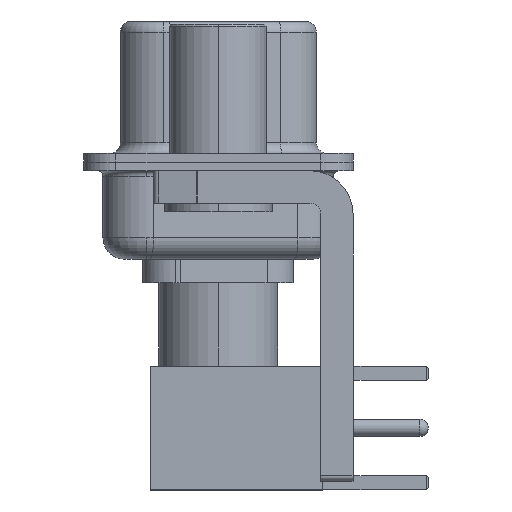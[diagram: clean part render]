
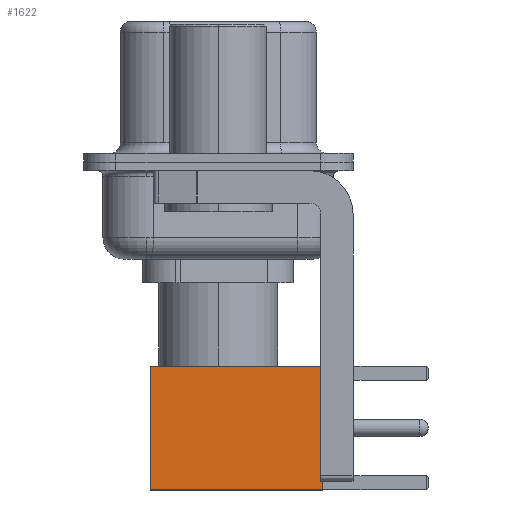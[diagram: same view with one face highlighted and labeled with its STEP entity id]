
A CAD part, left-side view. The second image highlights one B-rep face of the part: STEP entity #1622.
In plain terms, the highlighted face is planar.
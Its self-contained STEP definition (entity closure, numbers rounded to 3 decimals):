
#90 = ORIENTED_EDGE ( 'NONE', *, *, #21384, .F. ) ;
#355 = VERTEX_POINT ( 'NONE', #14789 ) ;
#576 = AXIS2_PLACEMENT_3D ( 'NONE', #3930, #20955, #12417 ) ;
#872 = CARTESIAN_POINT ( 'NONE',  ( -2.875, 2.875, 8. ) ) ;
#1123 = ORIENTED_EDGE ( 'NONE', *, *, #7999, .T. ) ;
#1265 = CARTESIAN_POINT ( 'NONE',  ( -2.875, 2.875, 0. ) ) ;
#1622 = ADVANCED_FACE ( 'NONE', ( #5616 ), #19503, .T. ) ;
#2827 = VECTOR ( 'NONE', #21003, 1000. ) ;
#3165 = CARTESIAN_POINT ( 'NONE',  ( 2.875, 2.875, 8. ) ) ;
#3533 = VERTEX_POINT ( 'NONE', #3165 ) ;
#3930 = CARTESIAN_POINT ( 'NONE',  ( 2.875, 2.875, 0. ) ) ;
#4391 = VERTEX_POINT ( 'NONE', #872 ) ;
#4683 = DIRECTION ( 'NONE',  ( -1., 0., 0. ) ) ;
#4715 = CARTESIAN_POINT ( 'NONE',  ( -2.875, 2.875, 0. ) ) ;
#5616 = FACE_OUTER_BOUND ( 'NONE', #14659, .T. ) ;
#6044 = LINE ( 'NONE', #6254, #14797 ) ;
#6254 = CARTESIAN_POINT ( 'NONE',  ( 0., 2.875, 8. ) ) ;
#6876 = CARTESIAN_POINT ( 'NONE',  ( 2.875, 2.875, 0. ) ) ;
#7000 = LINE ( 'NONE', #14170, #2827 ) ;
#7999 = EDGE_CURVE ( 'NONE', #355, #9861, #7000, .T. ) ;
#8033 = EDGE_CURVE ( 'NONE', #4391, #9861, #21232, .T. ) ;
#9861 = VERTEX_POINT ( 'NONE', #1265 ) ;
#10305 = VECTOR ( 'NONE', #13447, 1000. ) ;
#11564 = LINE ( 'NONE', #6876, #14530 ) ;
#12417 = DIRECTION ( 'NONE',  ( 0., 0., 1. ) ) ;
#12677 = EDGE_CURVE ( 'NONE', #3533, #355, #11564, .T. ) ;
#13447 = DIRECTION ( 'NONE',  ( 0., 0., -1. ) ) ;
#14170 = CARTESIAN_POINT ( 'NONE',  ( 0., 2.875, 0. ) ) ;
#14530 = VECTOR ( 'NONE', #20555, 1000. ) ;
#14659 = EDGE_LOOP ( 'NONE', ( #21612, #1123, #15480, #90 ) ) ;
#14789 = CARTESIAN_POINT ( 'NONE',  ( 2.875, 2.875, 0. ) ) ;
#14797 = VECTOR ( 'NONE', #4683, 1000. ) ;
#15480 = ORIENTED_EDGE ( 'NONE', *, *, #8033, .F. ) ;
#19503 = PLANE ( 'NONE',  #576 ) ;
#20555 = DIRECTION ( 'NONE',  ( 0., 0., -1. ) ) ;
#20955 = DIRECTION ( 'NONE',  ( 0., 1., 0. ) ) ;
#21003 = DIRECTION ( 'NONE',  ( -1., 0., 0. ) ) ;
#21232 = LINE ( 'NONE', #4715, #10305 ) ;
#21384 = EDGE_CURVE ( 'NONE', #3533, #4391, #6044, .T. ) ;
#21612 = ORIENTED_EDGE ( 'NONE', *, *, #12677, .T. ) ;
